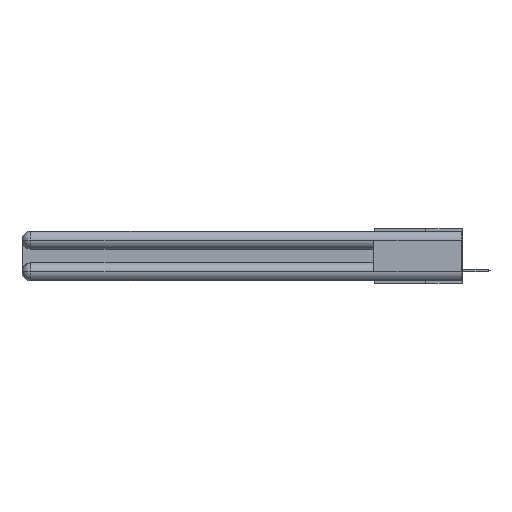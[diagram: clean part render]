
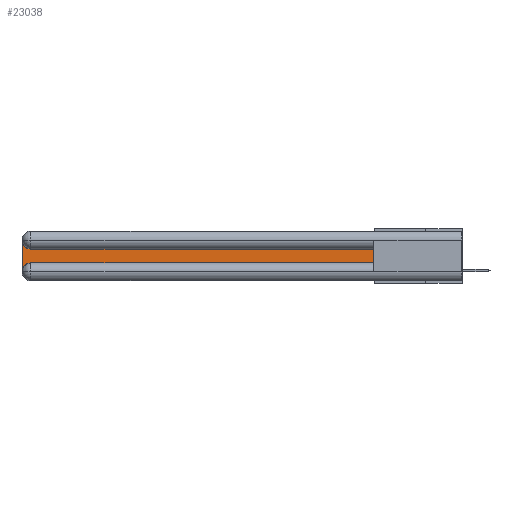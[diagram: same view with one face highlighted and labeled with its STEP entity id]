
A CAD part, left-side view. The second image highlights one B-rep face of the part: STEP entity #23038.
In plain terms, the highlighted planar face has unit normal (-1, 0, 0).
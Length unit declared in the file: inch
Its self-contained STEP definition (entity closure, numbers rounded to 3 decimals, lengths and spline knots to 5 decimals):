
#103 = CARTESIAN_POINT ( 'NONE',  ( 0.075, 0.6, -0.2175 ) ) ;
#822 = VERTEX_POINT ( 'NONE', #27526 ) ;
#1749 = LINE ( 'NONE', #5039, #20221 ) ;
#2178 = CARTESIAN_POINT ( 'NONE',  ( 0.075, 2.94, -0.2775 ) ) ;
#2665 = ORIENTED_EDGE ( 'NONE', *, *, #11203, .T. ) ;
#2726 = CARTESIAN_POINT ( 'NONE',  ( 0.075, 3., -0.0625 ) ) ;
#3873 = DIRECTION ( 'NONE',  ( 1., 0., 0. ) ) ;
#3987 = LINE ( 'NONE', #15353, #29802 ) ;
#4128 = ORIENTED_EDGE ( 'NONE', *, *, #17348, .T. ) ;
#4761 = CARTESIAN_POINT ( 'NONE',  ( 0.075, 3., -0.2775 ) ) ;
#5039 = CARTESIAN_POINT ( 'NONE',  ( 0.075, 3., -0.2175 ) ) ;
#5405 = ORIENTED_EDGE ( 'NONE', *, *, #15424, .T. ) ;
#6077 = CIRCLE ( 'NONE', #26511, 0.06 ) ;
#7455 = DIRECTION ( 'NONE',  ( 0., 0., -1. ) ) ;
#9096 = VERTEX_POINT ( 'NONE', #4761 ) ;
#10223 = DIRECTION ( 'NONE',  ( 1., 0., 0. ) ) ;
#11203 = EDGE_CURVE ( 'NONE', #9096, #15702, #6077, .T. ) ;
#11314 = VERTEX_POINT ( 'NONE', #2726 ) ;
#14762 = VECTOR ( 'NONE', #21644, 39.37008 ) ;
#15121 = DIRECTION ( 'NONE',  ( 1., 0., 0. ) ) ;
#15273 = CARTESIAN_POINT ( 'NONE',  ( 0.075, 3., -0.1225 ) ) ;
#15353 = CARTESIAN_POINT ( 'NONE',  ( 0.075, 0.6, -0.2175 ) ) ;
#15424 = EDGE_CURVE ( 'NONE', #15702, #24395, #3987, .T. ) ;
#15702 = VERTEX_POINT ( 'NONE', #16114 ) ;
#15924 = FACE_OUTER_BOUND ( 'NONE', #23523, .T. ) ;
#16114 = CARTESIAN_POINT ( 'NONE',  ( 0.075, 2.94, -0.2175 ) ) ;
#17348 = EDGE_CURVE ( 'NONE', #31069, #11314, #31432, .T. ) ;
#18646 = VECTOR ( 'NONE', #24744, 39.37008 ) ;
#19031 = CARTESIAN_POINT ( 'NONE',  ( 0.075, 0.6, -0.1225 ) ) ;
#19115 = CARTESIAN_POINT ( 'NONE',  ( 0.075, 2.94, -0.1225 ) ) ;
#20175 = EDGE_CURVE ( 'NONE', #24395, #822, #30542, .T. ) ;
#20205 = DIRECTION ( 'NONE',  ( 0., -1., 0. ) ) ;
#20221 = VECTOR ( 'NONE', #7455, 39.37008 ) ;
#21611 = AXIS2_PLACEMENT_3D ( 'NONE', #29989, #3873, #24835 ) ;
#21644 = DIRECTION ( 'NONE',  ( 0., 1., 0. ) ) ;
#22400 = PLANE ( 'NONE',  #33571 ) ;
#22565 = EDGE_CURVE ( 'NONE', #822, #31069, #28664, .T. ) ;
#23038 = ADVANCED_FACE ( 'NONE', ( #15924 ), #22400, .F. ) ;
#23405 = ORIENTED_EDGE ( 'NONE', *, *, #20175, .T. ) ;
#23523 = EDGE_LOOP ( 'NONE', ( #32270, #4128, #31350, #2665, #5405, #23405 ) ) ;
#23714 = EDGE_CURVE ( 'NONE', #11314, #9096, #1749, .T. ) ;
#24395 = VERTEX_POINT ( 'NONE', #103 ) ;
#24744 = DIRECTION ( 'NONE',  ( 0., 0., 1. ) ) ;
#24835 = DIRECTION ( 'NONE',  ( 0., 0., -1. ) ) ;
#26511 = AXIS2_PLACEMENT_3D ( 'NONE', #2178, #15121, #33440 ) ;
#27526 = CARTESIAN_POINT ( 'NONE',  ( 0.075, 0.6, -0.1225 ) ) ;
#28664 = LINE ( 'NONE', #19031, #14762 ) ;
#29802 = VECTOR ( 'NONE', #20205, 39.37008 ) ;
#29989 = CARTESIAN_POINT ( 'NONE',  ( 0.075, 2.94, -0.0625 ) ) ;
#30542 = LINE ( 'NONE', #32006, #18646 ) ;
#30969 = DIRECTION ( 'NONE',  ( 0., 0., -1. ) ) ;
#31069 = VERTEX_POINT ( 'NONE', #19115 ) ;
#31350 = ORIENTED_EDGE ( 'NONE', *, *, #23714, .T. ) ;
#31432 = CIRCLE ( 'NONE', #21611, 0.06 ) ;
#32006 = CARTESIAN_POINT ( 'NONE',  ( 0.075, 0.6, -0.2175 ) ) ;
#32270 = ORIENTED_EDGE ( 'NONE', *, *, #22565, .T. ) ;
#33440 = DIRECTION ( 'NONE',  ( 0., 0., -1. ) ) ;
#33571 = AXIS2_PLACEMENT_3D ( 'NONE', #15273, #10223, #30969 ) ;
